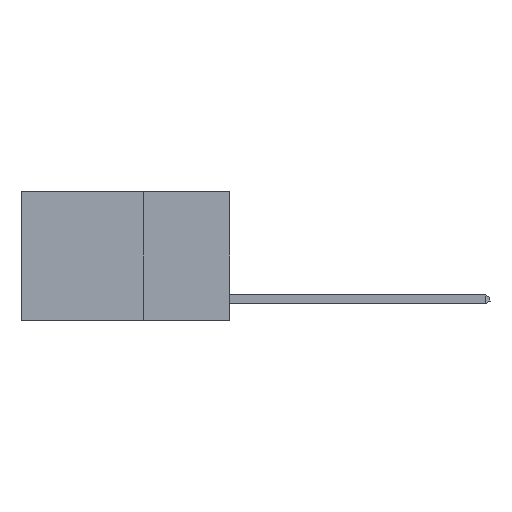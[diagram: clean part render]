
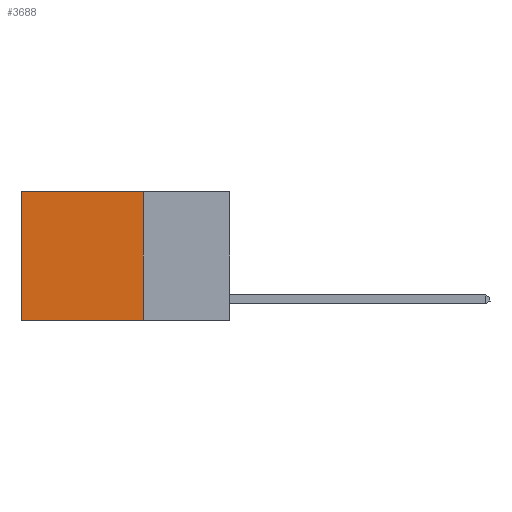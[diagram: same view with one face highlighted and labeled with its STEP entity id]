
A CAD part, left-side view. The second image highlights one B-rep face of the part: STEP entity #3688.
In plain terms, the highlighted planar face has unit normal (-1, 0, 0).
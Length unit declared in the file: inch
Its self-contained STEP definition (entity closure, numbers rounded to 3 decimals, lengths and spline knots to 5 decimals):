
#305 = PLANE ( 'NONE',  #4561 ) ;
#1723 = CARTESIAN_POINT ( 'NONE',  ( 0.2625, 0.25, 0. ) ) ;
#1759 = EDGE_CURVE ( 'NONE', #12658, #6219, #9100, .T. ) ;
#2342 = LINE ( 'NONE', #9324, #8806 ) ;
#3291 = DIRECTION ( 'NONE',  ( 0., 0., -1. ) ) ;
#3688 = ADVANCED_FACE ( 'NONE', ( #7563 ), #305, .F. ) ;
#4138 = EDGE_LOOP ( 'NONE', ( #10318, #5683, #4830, #15661 ) ) ;
#4559 = VECTOR ( 'NONE', #12481, 39.37008 ) ;
#4561 = AXIS2_PLACEMENT_3D ( 'NONE', #15490, #7284, #16838 ) ;
#4812 = DIRECTION ( 'NONE',  ( 0., 0., -1. ) ) ;
#4830 = ORIENTED_EDGE ( 'NONE', *, *, #5534, .F. ) ;
#4859 = VERTEX_POINT ( 'NONE', #16885 ) ;
#5197 = VECTOR ( 'NONE', #4812, 39.37008 ) ;
#5534 = EDGE_CURVE ( 'NONE', #12658, #8138, #14329, .T. ) ;
#5683 = ORIENTED_EDGE ( 'NONE', *, *, #5803, .F. ) ;
#5803 = EDGE_CURVE ( 'NONE', #8138, #4859, #2342, .T. ) ;
#6219 = VERTEX_POINT ( 'NONE', #11597 ) ;
#6640 = DIRECTION ( 'NONE',  ( 0., 1., 0. ) ) ;
#6982 = CARTESIAN_POINT ( 'NONE',  ( 0.2625, 0.25, 0. ) ) ;
#7284 = DIRECTION ( 'NONE',  ( 1., 0., 0. ) ) ;
#7563 = FACE_OUTER_BOUND ( 'NONE', #4138, .T. ) ;
#8138 = VERTEX_POINT ( 'NONE', #10151 ) ;
#8806 = VECTOR ( 'NONE', #6640, 39.37008 ) ;
#8810 = EDGE_CURVE ( 'NONE', #6219, #4859, #12499, .T. ) ;
#9100 = LINE ( 'NONE', #6982, #4559 ) ;
#9324 = CARTESIAN_POINT ( 'NONE',  ( 0.2625, 0.25, -0.37 ) ) ;
#10151 = CARTESIAN_POINT ( 'NONE',  ( 0.2625, 0.25, -0.37 ) ) ;
#10318 = ORIENTED_EDGE ( 'NONE', *, *, #8810, .T. ) ;
#11597 = CARTESIAN_POINT ( 'NONE',  ( 0.2625, 0.6, 0. ) ) ;
#12481 = DIRECTION ( 'NONE',  ( 0., 1., 0. ) ) ;
#12499 = LINE ( 'NONE', #15840, #5197 ) ;
#12658 = VERTEX_POINT ( 'NONE', #1723 ) ;
#14329 = LINE ( 'NONE', #15616, #17564 ) ;
#15490 = CARTESIAN_POINT ( 'NONE',  ( 0.2625, 0.25, 0. ) ) ;
#15616 = CARTESIAN_POINT ( 'NONE',  ( 0.2625, 0.25, 0. ) ) ;
#15661 = ORIENTED_EDGE ( 'NONE', *, *, #1759, .T. ) ;
#15840 = CARTESIAN_POINT ( 'NONE',  ( 0.2625, 0.6, 0. ) ) ;
#16838 = DIRECTION ( 'NONE',  ( 0., 0., -1. ) ) ;
#16885 = CARTESIAN_POINT ( 'NONE',  ( 0.2625, 0.6, -0.37 ) ) ;
#17564 = VECTOR ( 'NONE', #3291, 39.37008 ) ;
